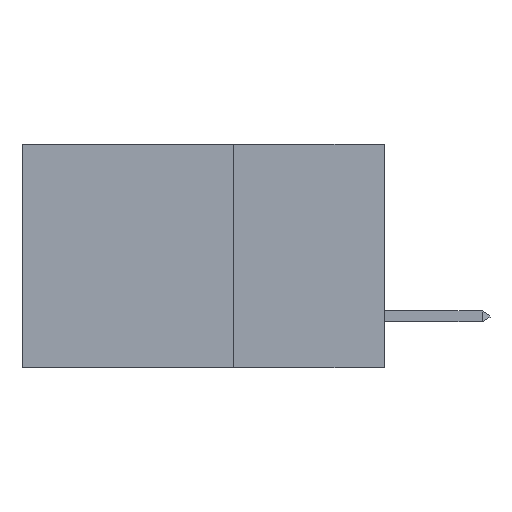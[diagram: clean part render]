
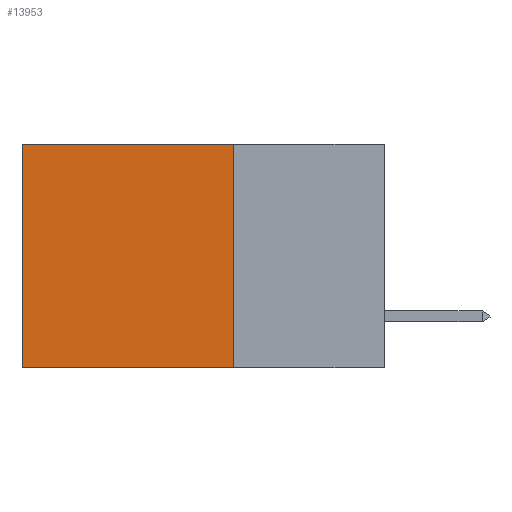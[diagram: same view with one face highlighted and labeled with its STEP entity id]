
A CAD part, left-side view. The second image highlights one B-rep face of the part: STEP entity #13953.
In plain terms, the highlighted planar face has unit normal (-1, 0, 0).
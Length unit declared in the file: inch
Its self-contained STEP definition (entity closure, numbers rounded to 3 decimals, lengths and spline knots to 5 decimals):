
#995 = CARTESIAN_POINT ( 'NONE',  ( 0.2875, 0.6, -0.37 ) ) ;
#2083 = EDGE_CURVE ( 'NONE', #18882, #20559, #13593, .T. ) ;
#2481 = EDGE_LOOP ( 'NONE', ( #8926, #16434, #13596, #19040 ) ) ;
#2845 = AXIS2_PLACEMENT_3D ( 'NONE', #20904, #22875, #11010 ) ;
#3465 = DIRECTION ( 'NONE',  ( 0., 1., 0. ) ) ;
#6113 = DIRECTION ( 'NONE',  ( 0., 0., -1. ) ) ;
#6497 = CARTESIAN_POINT ( 'NONE',  ( 0.2875, 0.25, -0.37 ) ) ;
#6602 = CARTESIAN_POINT ( 'NONE',  ( 0.2875, 0.25, 0. ) ) ;
#6948 = PLANE ( 'NONE',  #2845 ) ;
#7587 = EDGE_CURVE ( 'NONE', #18882, #10670, #14385, .T. ) ;
#7890 = VERTEX_POINT ( 'NONE', #995 ) ;
#8926 = ORIENTED_EDGE ( 'NONE', *, *, #16117, .T. ) ;
#9887 = VECTOR ( 'NONE', #3465, 39.37008 ) ;
#10201 = CARTESIAN_POINT ( 'NONE',  ( 0.2875, 0.6, 0. ) ) ;
#10259 = DIRECTION ( 'NONE',  ( 0., 1., 0. ) ) ;
#10670 = VERTEX_POINT ( 'NONE', #12020 ) ;
#11010 = DIRECTION ( 'NONE',  ( 0., 0., -1. ) ) ;
#12020 = CARTESIAN_POINT ( 'NONE',  ( 0.2875, 0.6, 0. ) ) ;
#12297 = CARTESIAN_POINT ( 'NONE',  ( 0.2875, 0.25, 0. ) ) ;
#12773 = FACE_OUTER_BOUND ( 'NONE', #2481, .T. ) ;
#13108 = CARTESIAN_POINT ( 'NONE',  ( 0.2875, 0.25, 0. ) ) ;
#13593 = LINE ( 'NONE', #6602, #23507 ) ;
#13596 = ORIENTED_EDGE ( 'NONE', *, *, #2083, .F. ) ;
#13953 = ADVANCED_FACE ( 'NONE', ( #12773 ), #6948, .F. ) ;
#14385 = LINE ( 'NONE', #12297, #24292 ) ;
#14656 = EDGE_CURVE ( 'NONE', #20559, #7890, #20477, .T. ) ;
#16117 = EDGE_CURVE ( 'NONE', #10670, #7890, #24223, .T. ) ;
#16434 = ORIENTED_EDGE ( 'NONE', *, *, #14656, .F. ) ;
#17626 = CARTESIAN_POINT ( 'NONE',  ( 0.2875, 0.25, -0.37 ) ) ;
#18882 = VERTEX_POINT ( 'NONE', #13108 ) ;
#19040 = ORIENTED_EDGE ( 'NONE', *, *, #7587, .T. ) ;
#19580 = VECTOR ( 'NONE', #24105, 39.37008 ) ;
#20477 = LINE ( 'NONE', #17626, #9887 ) ;
#20559 = VERTEX_POINT ( 'NONE', #6497 ) ;
#20904 = CARTESIAN_POINT ( 'NONE',  ( 0.2875, 0.25, 0. ) ) ;
#22875 = DIRECTION ( 'NONE',  ( 1., 0., 0. ) ) ;
#23507 = VECTOR ( 'NONE', #6113, 39.37008 ) ;
#24105 = DIRECTION ( 'NONE',  ( 0., 0., -1. ) ) ;
#24223 = LINE ( 'NONE', #10201, #19580 ) ;
#24292 = VECTOR ( 'NONE', #10259, 39.37008 ) ;
